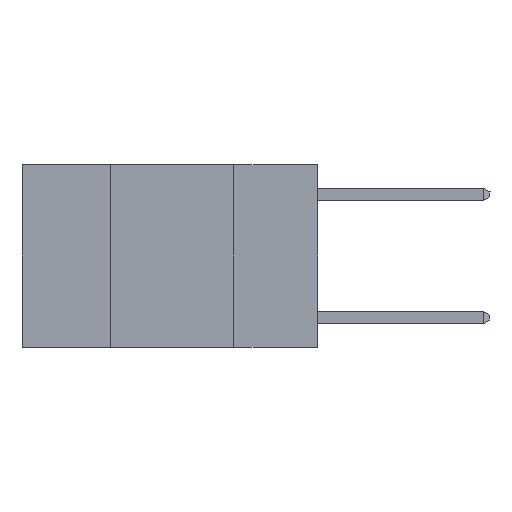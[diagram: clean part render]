
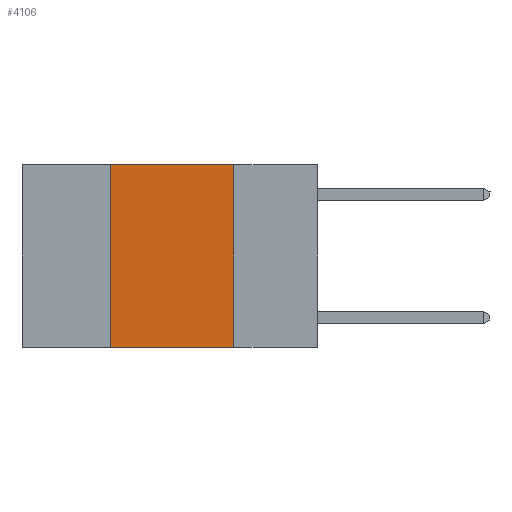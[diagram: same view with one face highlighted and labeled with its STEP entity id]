
A CAD part, left-side view. The second image highlights one B-rep face of the part: STEP entity #4106.
In plain terms, the highlighted planar face has unit normal (-1, 0, 0).
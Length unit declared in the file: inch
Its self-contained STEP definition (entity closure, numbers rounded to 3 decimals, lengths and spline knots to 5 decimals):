
#486 = DIRECTION ( 'NONE',  ( 0., -1., 0. ) ) ;
#661 = EDGE_CURVE ( 'NONE', #2386, #11566, #1008, .T. ) ;
#868 = DIRECTION ( 'NONE',  ( 0., 0., -1. ) ) ;
#912 = DIRECTION ( 'NONE',  ( 0., -1., 0. ) ) ;
#967 = CARTESIAN_POINT ( 'NONE',  ( 0., 0.42, 0. ) ) ;
#1008 = LINE ( 'NONE', #9514, #5738 ) ;
#1268 = DIRECTION ( 'NONE',  ( 0., 0., 1. ) ) ;
#1412 = EDGE_LOOP ( 'NONE', ( #9537, #10175, #6531, #6762 ) ) ;
#1677 = FACE_OUTER_BOUND ( 'NONE', #1412, .T. ) ;
#2386 = VERTEX_POINT ( 'NONE', #8279 ) ;
#3312 = EDGE_CURVE ( 'NONE', #3805, #2386, #4720, .T. ) ;
#3337 = CARTESIAN_POINT ( 'NONE',  ( 0., 0.42, 0. ) ) ;
#3357 = AXIS2_PLACEMENT_3D ( 'NONE', #11565, #9696, #868 ) ;
#3805 = VERTEX_POINT ( 'NONE', #967 ) ;
#4102 = LINE ( 'NONE', #8394, #11454 ) ;
#4106 = ADVANCED_FACE ( 'NONE', ( #1677 ), #12470, .F. ) ;
#4225 = CARTESIAN_POINT ( 'NONE',  ( 0., 0.17, -0.37 ) ) ;
#4720 = LINE ( 'NONE', #7179, #9568 ) ;
#4893 = EDGE_CURVE ( 'NONE', #7153, #3805, #9769, .T. ) ;
#5738 = VECTOR ( 'NONE', #6997, 39.37008 ) ;
#6531 = ORIENTED_EDGE ( 'NONE', *, *, #4893, .F. ) ;
#6722 = CARTESIAN_POINT ( 'NONE',  ( 0., 0.42, -0.37 ) ) ;
#6762 = ORIENTED_EDGE ( 'NONE', *, *, #7653, .T. ) ;
#6997 = DIRECTION ( 'NONE',  ( 0., 0., -1. ) ) ;
#7153 = VERTEX_POINT ( 'NONE', #6722 ) ;
#7179 = CARTESIAN_POINT ( 'NONE',  ( 0., 0.6, 0. ) ) ;
#7653 = EDGE_CURVE ( 'NONE', #7153, #11566, #4102, .T. ) ;
#8279 = CARTESIAN_POINT ( 'NONE',  ( 0., 0.17, 0. ) ) ;
#8394 = CARTESIAN_POINT ( 'NONE',  ( 0., 0.6, -0.37 ) ) ;
#9457 = VECTOR ( 'NONE', #1268, 39.37008 ) ;
#9514 = CARTESIAN_POINT ( 'NONE',  ( 0., 0.17, 0. ) ) ;
#9537 = ORIENTED_EDGE ( 'NONE', *, *, #661, .F. ) ;
#9568 = VECTOR ( 'NONE', #912, 39.37008 ) ;
#9696 = DIRECTION ( 'NONE',  ( 1., 0., 0. ) ) ;
#9769 = LINE ( 'NONE', #3337, #9457 ) ;
#10175 = ORIENTED_EDGE ( 'NONE', *, *, #3312, .F. ) ;
#11454 = VECTOR ( 'NONE', #486, 39.37008 ) ;
#11565 = CARTESIAN_POINT ( 'NONE',  ( 0., 0.6, 0. ) ) ;
#11566 = VERTEX_POINT ( 'NONE', #4225 ) ;
#12470 = PLANE ( 'NONE',  #3357 ) ;
